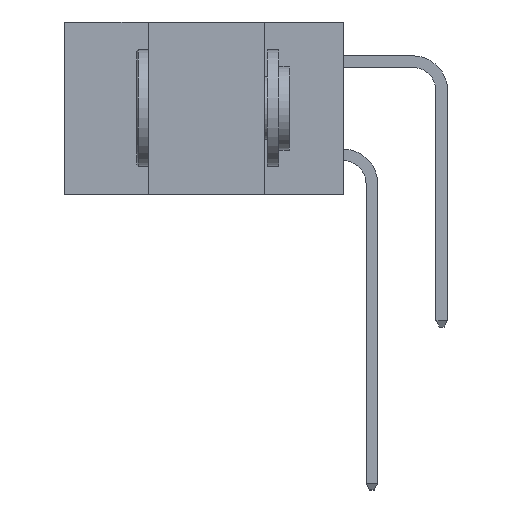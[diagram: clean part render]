
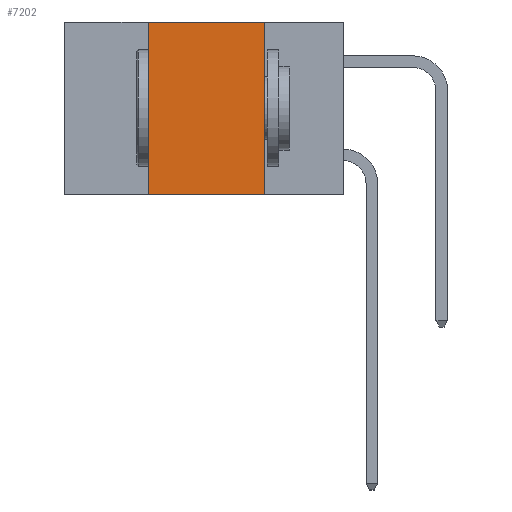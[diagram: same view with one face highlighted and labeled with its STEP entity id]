
A CAD part, left-side view. The second image highlights one B-rep face of the part: STEP entity #7202.
In plain terms, the highlighted planar face has unit normal (-1, 0, 0).
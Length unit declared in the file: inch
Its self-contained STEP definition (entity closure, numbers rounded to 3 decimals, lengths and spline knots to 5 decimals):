
#1501 = ORIENTED_EDGE ( 'NONE', *, *, #7387, .F. ) ;
#2441 = DIRECTION ( 'NONE',  ( 0., 0., 1. ) ) ;
#3390 = LINE ( 'NONE', #5579, #11644 ) ;
#3519 = CARTESIAN_POINT ( 'NONE',  ( 0., 0.17, 0. ) ) ;
#5119 = VECTOR ( 'NONE', #10502, 39.37008 ) ;
#5352 = EDGE_CURVE ( 'NONE', #7601, #11608, #3390, .T. ) ;
#5579 = CARTESIAN_POINT ( 'NONE',  ( 0., 0.6, 0. ) ) ;
#5655 = CARTESIAN_POINT ( 'NONE',  ( 0., 0.42, -0.37 ) ) ;
#6595 = ORIENTED_EDGE ( 'NONE', *, *, #20775, .F. ) ;
#6789 = CARTESIAN_POINT ( 'NONE',  ( 0., 0.6, 0. ) ) ;
#7199 = LINE ( 'NONE', #7571, #15523 ) ;
#7202 = ADVANCED_FACE ( 'NONE', ( #16287 ), #16723, .F. ) ;
#7387 = EDGE_CURVE ( 'NONE', #11566, #7601, #17062, .T. ) ;
#7571 = CARTESIAN_POINT ( 'NONE',  ( 0., 0.6, -0.37 ) ) ;
#7601 = VERTEX_POINT ( 'NONE', #11881 ) ;
#8464 = DIRECTION ( 'NONE',  ( 0., 0., -1. ) ) ;
#8844 = CARTESIAN_POINT ( 'NONE',  ( 0., 0.17, -0.37 ) ) ;
#9259 = EDGE_LOOP ( 'NONE', ( #6595, #18035, #1501, #11291 ) ) ;
#10015 = LINE ( 'NONE', #8844, #5119 ) ;
#10238 = VERTEX_POINT ( 'NONE', #16774 ) ;
#10502 = DIRECTION ( 'NONE',  ( 0., 0., -1. ) ) ;
#11291 = ORIENTED_EDGE ( 'NONE', *, *, #14709, .T. ) ;
#11566 = VERTEX_POINT ( 'NONE', #13253 ) ;
#11608 = VERTEX_POINT ( 'NONE', #3519 ) ;
#11644 = VECTOR ( 'NONE', #12171, 39.37008 ) ;
#11881 = CARTESIAN_POINT ( 'NONE',  ( 0., 0.42, 0. ) ) ;
#12171 = DIRECTION ( 'NONE',  ( 0., -1., 0. ) ) ;
#12669 = VECTOR ( 'NONE', #2441, 39.37008 ) ;
#13253 = CARTESIAN_POINT ( 'NONE',  ( 0., 0.42, -0.37 ) ) ;
#14709 = EDGE_CURVE ( 'NONE', #11566, #10238, #7199, .T. ) ;
#14929 = AXIS2_PLACEMENT_3D ( 'NONE', #6789, #18401, #8464 ) ;
#15523 = VECTOR ( 'NONE', #19177, 39.37008 ) ;
#16287 = FACE_OUTER_BOUND ( 'NONE', #9259, .T. ) ;
#16723 = PLANE ( 'NONE',  #14929 ) ;
#16774 = CARTESIAN_POINT ( 'NONE',  ( 0., 0.17, -0.37 ) ) ;
#17062 = LINE ( 'NONE', #5655, #12669 ) ;
#18035 = ORIENTED_EDGE ( 'NONE', *, *, #5352, .F. ) ;
#18401 = DIRECTION ( 'NONE',  ( 1., 0., 0. ) ) ;
#19177 = DIRECTION ( 'NONE',  ( 0., -1., 0. ) ) ;
#20775 = EDGE_CURVE ( 'NONE', #11608, #10238, #10015, .T. ) ;
